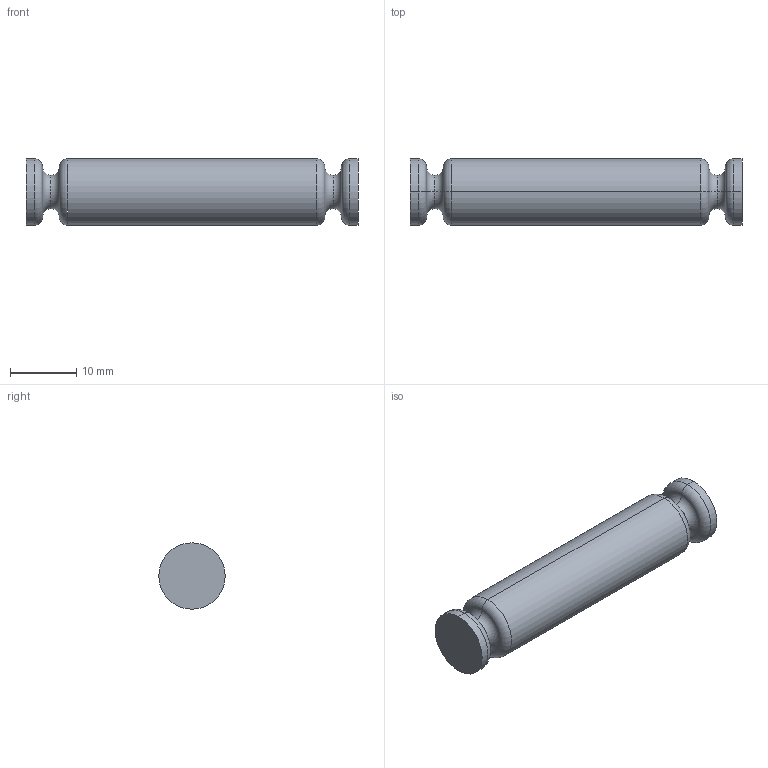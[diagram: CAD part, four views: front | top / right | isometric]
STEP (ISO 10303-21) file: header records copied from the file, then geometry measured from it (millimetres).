
FILE_DESCRIPTION (( 'STEP AP203' ), '1' );
FILE_NAME ('Long_Hammer_Slide_Pin.STEP', '2013-11-14T05:09:22', ( '' ), ( '' ), 'SwSTEP 2.0', 'SolidWorks 2013', '' );
FILE_SCHEMA (( 'CONFIG_CONTROL_DESIGN' ));
Length unit declared in the file: millimetre
Products named in the file (1): Long_Hammer_Slide_Pin
Bounding box: 50 x 10 x 10 mm (x, y, z)
Volume: 3616.1 mm3; surface area: 1783.8 mm2
Topology: 1 solids, 1 shells, 24 faces, 46 edges, 24 vertices
Faces by surface type: torus 16, cylinder 6, plane 2
Entity records: 687 total; most frequent: DIRECTION 136, CARTESIAN_POINT 95, ORIENTED_EDGE 92, AXIS2_PLACEMENT_3D 65, EDGE_CURVE 46, CIRCLE 40, EDGE_LOOP 24, FACE_OUTER_BOUND 24
